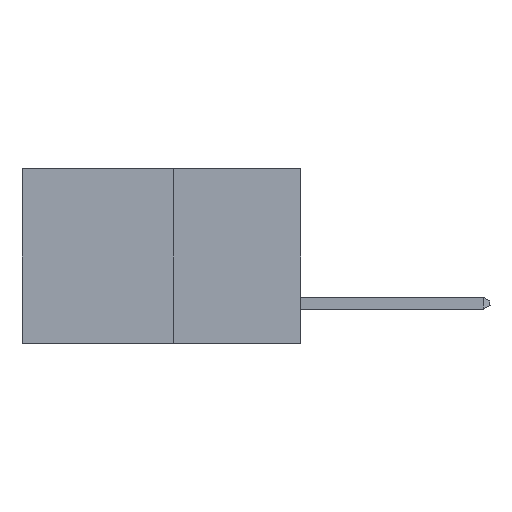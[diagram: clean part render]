
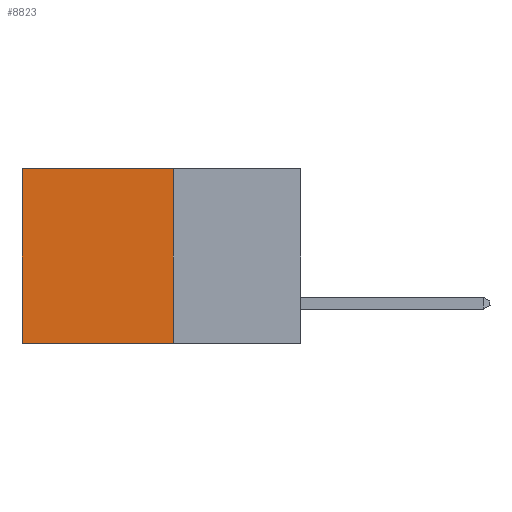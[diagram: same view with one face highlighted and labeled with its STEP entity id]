
A CAD part, left-side view. The second image highlights one B-rep face of the part: STEP entity #8823.
In plain terms, the highlighted planar face has unit normal (-1, 0, 0).
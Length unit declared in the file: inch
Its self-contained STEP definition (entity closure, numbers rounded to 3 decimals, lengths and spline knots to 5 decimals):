
#129 = VERTEX_POINT ( 'NONE', #8924 ) ;
#202 = VECTOR ( 'NONE', #7812, 39.37008 ) ;
#714 = LINE ( 'NONE', #7521, #9403 ) ;
#752 = VERTEX_POINT ( 'NONE', #11239 ) ;
#987 = CARTESIAN_POINT ( 'NONE',  ( 0.277, 0.27, 0. ) ) ;
#1067 = EDGE_CURVE ( 'NONE', #8761, #9788, #3043, .T. ) ;
#2981 = VECTOR ( 'NONE', #13436, 39.37008 ) ;
#3043 = LINE ( 'NONE', #12797, #202 ) ;
#3945 = EDGE_CURVE ( 'NONE', #752, #129, #8526, .T. ) ;
#4197 = DIRECTION ( 'NONE',  ( 0., 1., 0. ) ) ;
#4291 = EDGE_LOOP ( 'NONE', ( #6452, #6466, #11515, #11603 ) ) ;
#4871 = VECTOR ( 'NONE', #8919, 39.37008 ) ;
#5353 = DIRECTION ( 'NONE',  ( 1., 0., 0. ) ) ;
#6452 = ORIENTED_EDGE ( 'NONE', *, *, #3945, .T. ) ;
#6466 = ORIENTED_EDGE ( 'NONE', *, *, #12865, .F. ) ;
#7521 = CARTESIAN_POINT ( 'NONE',  ( 0.277, 0.27, -0.37 ) ) ;
#7812 = DIRECTION ( 'NONE',  ( 0., 0., -1. ) ) ;
#8526 = LINE ( 'NONE', #12948, #2981 ) ;
#8761 = VERTEX_POINT ( 'NONE', #13655 ) ;
#8823 = ADVANCED_FACE ( 'NONE', ( #11579 ), #11685, .F. ) ;
#8919 = DIRECTION ( 'NONE',  ( 0., 1., 0. ) ) ;
#8924 = CARTESIAN_POINT ( 'NONE',  ( 0.277, 0.59, -0.37 ) ) ;
#9403 = VECTOR ( 'NONE', #4197, 39.37008 ) ;
#9788 = VERTEX_POINT ( 'NONE', #11569 ) ;
#10064 = AXIS2_PLACEMENT_3D ( 'NONE', #10653, #5353, #12743 ) ;
#10234 = LINE ( 'NONE', #987, #4871 ) ;
#10653 = CARTESIAN_POINT ( 'NONE',  ( 0.277, 0.27, -0.37 ) ) ;
#11239 = CARTESIAN_POINT ( 'NONE',  ( 0.277, 0.59, 0. ) ) ;
#11267 = EDGE_CURVE ( 'NONE', #8761, #752, #10234, .T. ) ;
#11515 = ORIENTED_EDGE ( 'NONE', *, *, #1067, .F. ) ;
#11569 = CARTESIAN_POINT ( 'NONE',  ( 0.277, 0.27, -0.37 ) ) ;
#11579 = FACE_OUTER_BOUND ( 'NONE', #4291, .T. ) ;
#11603 = ORIENTED_EDGE ( 'NONE', *, *, #11267, .T. ) ;
#11685 = PLANE ( 'NONE',  #10064 ) ;
#12743 = DIRECTION ( 'NONE',  ( 0., 0., -1. ) ) ;
#12797 = CARTESIAN_POINT ( 'NONE',  ( 0.277, 0.27, -0.37 ) ) ;
#12865 = EDGE_CURVE ( 'NONE', #9788, #129, #714, .T. ) ;
#12948 = CARTESIAN_POINT ( 'NONE',  ( 0.277, 0.59, -0.37 ) ) ;
#13436 = DIRECTION ( 'NONE',  ( 0., 0., -1. ) ) ;
#13655 = CARTESIAN_POINT ( 'NONE',  ( 0.277, 0.27, 0. ) ) ;
